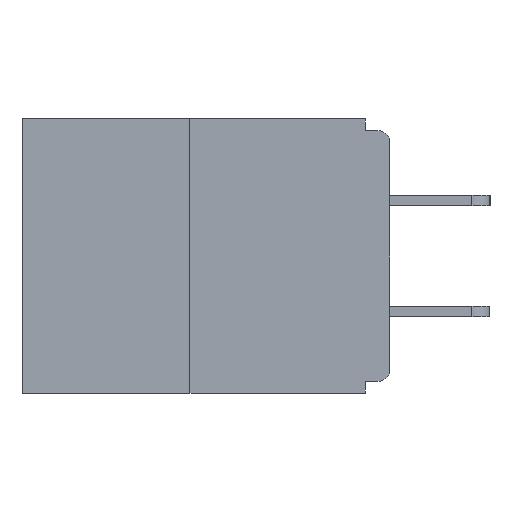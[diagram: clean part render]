
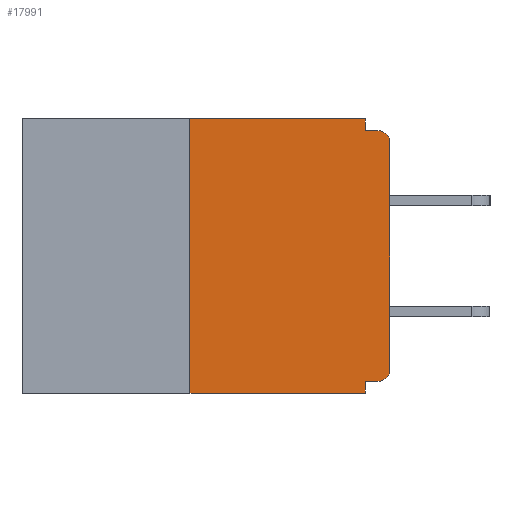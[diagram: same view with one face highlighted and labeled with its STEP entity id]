
A CAD part, left-side view. The second image highlights one B-rep face of the part: STEP entity #17991.
In plain terms, the highlighted planar face has unit normal (-1, 0, 0).
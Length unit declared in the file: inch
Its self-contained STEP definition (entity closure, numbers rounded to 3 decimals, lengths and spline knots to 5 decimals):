
#201 = EDGE_CURVE ( 'NONE', #11185, #7076, #11614, .T. ) ;
#217 = ORIENTED_EDGE ( 'NONE', *, *, #15198, .F. ) ;
#758 = CARTESIAN_POINT ( 'NONE',  ( 0., 0.015, -0.03 ) ) ;
#769 = VERTEX_POINT ( 'NONE', #11656 ) ;
#999 = AXIS2_PLACEMENT_3D ( 'NONE', #5440, #11258, #9733 ) ;
#1139 = FACE_OUTER_BOUND ( 'NONE', #9064, .T. ) ;
#1377 = DIRECTION ( 'NONE',  ( 0., 1., 0. ) ) ;
#1438 = CIRCLE ( 'NONE', #16701, 0.015 ) ;
#1461 = VERTEX_POINT ( 'NONE', #15515 ) ;
#1500 = DIRECTION ( 'NONE',  ( 0., 0., 1. ) ) ;
#2039 = ORIENTED_EDGE ( 'NONE', *, *, #11858, .T. ) ;
#2107 = LINE ( 'NONE', #16837, #6714 ) ;
#2603 = ORIENTED_EDGE ( 'NONE', *, *, #16148, .F. ) ;
#2707 = VECTOR ( 'NONE', #2786, 39.37008 ) ;
#2786 = DIRECTION ( 'NONE',  ( 0., 0., -1. ) ) ;
#3021 = DIRECTION ( 'NONE',  ( 0., 0., 1. ) ) ;
#3038 = VERTEX_POINT ( 'NONE', #3112 ) ;
#3112 = CARTESIAN_POINT ( 'NONE',  ( 0., 0.015, -0.015 ) ) ;
#3181 = VERTEX_POINT ( 'NONE', #8065 ) ;
#3570 = ORIENTED_EDGE ( 'NONE', *, *, #7579, .F. ) ;
#4077 = DIRECTION ( 'NONE',  ( 0., 0., -1. ) ) ;
#4090 = LINE ( 'NONE', #5510, #18612 ) ;
#4153 = DIRECTION ( 'NONE',  ( -1., 0., 0. ) ) ;
#4249 = VECTOR ( 'NONE', #6362, 39.37008 ) ;
#4330 = LINE ( 'NONE', #5856, #2707 ) ;
#5440 = CARTESIAN_POINT ( 'NONE',  ( 0., 0.46, 0. ) ) ;
#5499 = CARTESIAN_POINT ( 'NONE',  ( 0., 0.031, 0. ) ) ;
#5510 = CARTESIAN_POINT ( 'NONE',  ( 0., 0.25, 0. ) ) ;
#5628 = PLANE ( 'NONE',  #999 ) ;
#5856 = CARTESIAN_POINT ( 'NONE',  ( 0., 0.031, -0.343 ) ) ;
#5950 = VERTEX_POINT ( 'NONE', #10111 ) ;
#6362 = DIRECTION ( 'NONE',  ( 0., -1., 0. ) ) ;
#6394 = EDGE_CURVE ( 'NONE', #3181, #12018, #7608, .T. ) ;
#6424 = ORIENTED_EDGE ( 'NONE', *, *, #201, .F. ) ;
#6452 = CARTESIAN_POINT ( 'NONE',  ( 0., 0.46, 0. ) ) ;
#6586 = DIRECTION ( 'NONE',  ( -1., 0., 0. ) ) ;
#6589 = ORIENTED_EDGE ( 'NONE', *, *, #6394, .T. ) ;
#6714 = VECTOR ( 'NONE', #9569, 39.37008 ) ;
#7076 = VERTEX_POINT ( 'NONE', #15407 ) ;
#7292 = DIRECTION ( 'NONE',  ( 0., 0., -1. ) ) ;
#7465 = CARTESIAN_POINT ( 'NONE',  ( 0., 0.031, 0. ) ) ;
#7579 = EDGE_CURVE ( 'NONE', #5950, #769, #4090, .T. ) ;
#7608 = LINE ( 'NONE', #14810, #15984 ) ;
#7806 = EDGE_CURVE ( 'NONE', #5950, #12341, #15365, .T. ) ;
#8065 = CARTESIAN_POINT ( 'NONE',  ( 0., 0., -0.313 ) ) ;
#8096 = DIRECTION ( 'NONE',  ( 0., 0., -1. ) ) ;
#9064 = EDGE_LOOP ( 'NONE', ( #9960, #3570, #10442, #2603, #12300, #2039, #6589, #10759, #217, #6424 ) ) ;
#9569 = DIRECTION ( 'NONE',  ( 0., -1., 0. ) ) ;
#9614 = DIRECTION ( 'NONE',  ( 0., -1., 0. ) ) ;
#9733 = DIRECTION ( 'NONE',  ( 0., 0., -1. ) ) ;
#9871 = LINE ( 'NONE', #14200, #17577 ) ;
#9960 = ORIENTED_EDGE ( 'NONE', *, *, #15809, .F. ) ;
#10028 = EDGE_CURVE ( 'NONE', #12018, #3038, #15605, .T. ) ;
#10110 = AXIS2_PLACEMENT_3D ( 'NONE', #758, #6586, #8096 ) ;
#10111 = CARTESIAN_POINT ( 'NONE',  ( 0., 0.25, -0.343 ) ) ;
#10442 = ORIENTED_EDGE ( 'NONE', *, *, #7806, .T. ) ;
#10474 = LINE ( 'NONE', #6452, #4249 ) ;
#10536 = EDGE_CURVE ( 'NONE', #13769, #1461, #9871, .T. ) ;
#10759 = ORIENTED_EDGE ( 'NONE', *, *, #10028, .T. ) ;
#11185 = VERTEX_POINT ( 'NONE', #7465 ) ;
#11258 = DIRECTION ( 'NONE',  ( 1., 0., 0. ) ) ;
#11386 = CARTESIAN_POINT ( 'NONE',  ( 0., 0.031, -0.343 ) ) ;
#11614 = LINE ( 'NONE', #5499, #15881 ) ;
#11656 = CARTESIAN_POINT ( 'NONE',  ( 0., 0.25, 0. ) ) ;
#11858 = EDGE_CURVE ( 'NONE', #13769, #3181, #1438, .T. ) ;
#12018 = VERTEX_POINT ( 'NONE', #17911 ) ;
#12204 = CARTESIAN_POINT ( 'NONE',  ( 0., 0.46, -0.343 ) ) ;
#12300 = ORIENTED_EDGE ( 'NONE', *, *, #10536, .F. ) ;
#12341 = VERTEX_POINT ( 'NONE', #11386 ) ;
#12537 = VECTOR ( 'NONE', #9614, 39.37008 ) ;
#13769 = VERTEX_POINT ( 'NONE', #15125 ) ;
#14200 = CARTESIAN_POINT ( 'NONE',  ( 0., 0., -0.328 ) ) ;
#14810 = CARTESIAN_POINT ( 'NONE',  ( 0., 0., 0. ) ) ;
#15125 = CARTESIAN_POINT ( 'NONE',  ( 0., 0.015, -0.328 ) ) ;
#15198 = EDGE_CURVE ( 'NONE', #7076, #3038, #2107, .T. ) ;
#15365 = LINE ( 'NONE', #12204, #12537 ) ;
#15407 = CARTESIAN_POINT ( 'NONE',  ( 0., 0.031, -0.015 ) ) ;
#15515 = CARTESIAN_POINT ( 'NONE',  ( 0., 0.031, -0.328 ) ) ;
#15605 = CIRCLE ( 'NONE', #10110, 0.015 ) ;
#15809 = EDGE_CURVE ( 'NONE', #769, #11185, #10474, .T. ) ;
#15881 = VECTOR ( 'NONE', #4077, 39.37008 ) ;
#15984 = VECTOR ( 'NONE', #3021, 39.37008 ) ;
#16148 = EDGE_CURVE ( 'NONE', #1461, #12341, #4330, .T. ) ;
#16701 = AXIS2_PLACEMENT_3D ( 'NONE', #17538, #4153, #7292 ) ;
#16837 = CARTESIAN_POINT ( 'NONE',  ( 0., 0., -0.015 ) ) ;
#17538 = CARTESIAN_POINT ( 'NONE',  ( 0., 0.015, -0.313 ) ) ;
#17577 = VECTOR ( 'NONE', #1377, 39.37008 ) ;
#17911 = CARTESIAN_POINT ( 'NONE',  ( 0., 0., -0.03 ) ) ;
#17991 = ADVANCED_FACE ( 'NONE', ( #1139 ), #5628, .F. ) ;
#18612 = VECTOR ( 'NONE', #1500, 39.37008 ) ;
